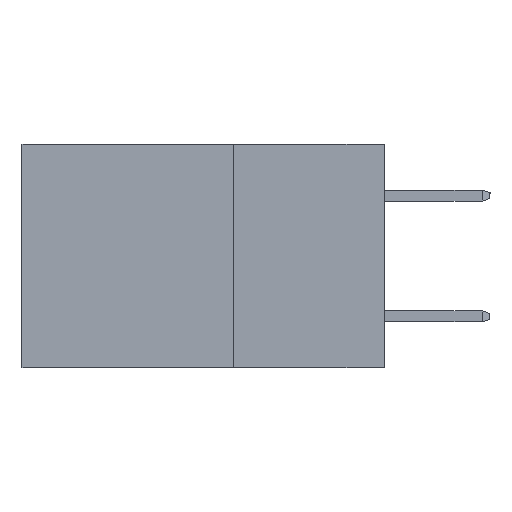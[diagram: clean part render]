
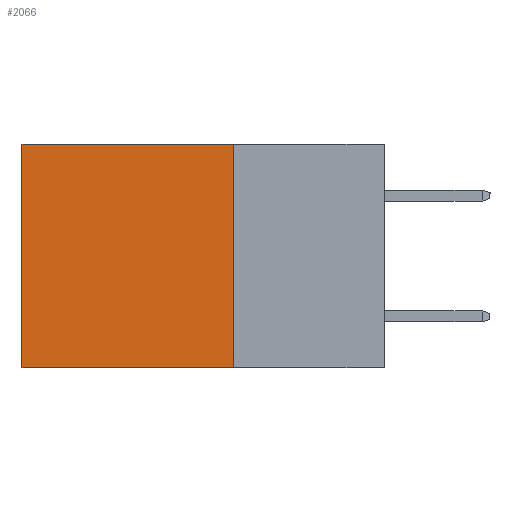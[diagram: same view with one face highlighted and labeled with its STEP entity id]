
A CAD part, left-side view. The second image highlights one B-rep face of the part: STEP entity #2066.
In plain terms, the highlighted planar face has unit normal (-1, 0, 0).
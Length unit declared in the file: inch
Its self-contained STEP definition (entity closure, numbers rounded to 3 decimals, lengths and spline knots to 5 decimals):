
#431 = DIRECTION ( 'NONE',  ( 0., 0., -1. ) ) ;
#452 = AXIS2_PLACEMENT_3D ( 'NONE', #2408, #16525, #431 ) ;
#530 = VERTEX_POINT ( 'NONE', #1109 ) ;
#1109 = CARTESIAN_POINT ( 'NONE',  ( 0.2615, 0.6, 0. ) ) ;
#1752 = ORIENTED_EDGE ( 'NONE', *, *, #14193, .F. ) ;
#2066 = ADVANCED_FACE ( 'NONE', ( #13280 ), #18518, .F. ) ;
#2239 = ORIENTED_EDGE ( 'NONE', *, *, #2568, .T. ) ;
#2408 = CARTESIAN_POINT ( 'NONE',  ( 0.2615, 0.25, -0.37 ) ) ;
#2432 = CARTESIAN_POINT ( 'NONE',  ( 0.2615, 0.25, 0. ) ) ;
#2568 = EDGE_CURVE ( 'NONE', #530, #4409, #3972, .T. ) ;
#3095 = VECTOR ( 'NONE', #10086, 39.37008 ) ;
#3418 = LINE ( 'NONE', #11703, #9938 ) ;
#3870 = LINE ( 'NONE', #7281, #6045 ) ;
#3972 = LINE ( 'NONE', #20282, #5568 ) ;
#4409 = VERTEX_POINT ( 'NONE', #16018 ) ;
#5230 = CARTESIAN_POINT ( 'NONE',  ( 0.2615, 0.25, 0. ) ) ;
#5539 = EDGE_CURVE ( 'NONE', #17838, #14682, #3870, .T. ) ;
#5568 = VECTOR ( 'NONE', #12243, 39.37008 ) ;
#6045 = VECTOR ( 'NONE', #7177, 39.37008 ) ;
#7177 = DIRECTION ( 'NONE',  ( 0., 0., -1. ) ) ;
#7281 = CARTESIAN_POINT ( 'NONE',  ( 0.2615, 0.25, -0.37 ) ) ;
#8036 = DIRECTION ( 'NONE',  ( 0., 1., 0. ) ) ;
#8759 = ORIENTED_EDGE ( 'NONE', *, *, #19135, .T. ) ;
#9938 = VECTOR ( 'NONE', #8036, 39.37008 ) ;
#10048 = CARTESIAN_POINT ( 'NONE',  ( 0.2615, 0.25, -0.37 ) ) ;
#10086 = DIRECTION ( 'NONE',  ( 0., 1., 0. ) ) ;
#11703 = CARTESIAN_POINT ( 'NONE',  ( 0.2615, 0.25, -0.37 ) ) ;
#12243 = DIRECTION ( 'NONE',  ( 0., 0., -1. ) ) ;
#13280 = FACE_OUTER_BOUND ( 'NONE', #19940, .T. ) ;
#14193 = EDGE_CURVE ( 'NONE', #14682, #4409, #3418, .T. ) ;
#14682 = VERTEX_POINT ( 'NONE', #10048 ) ;
#16018 = CARTESIAN_POINT ( 'NONE',  ( 0.2615, 0.6, -0.37 ) ) ;
#16423 = ORIENTED_EDGE ( 'NONE', *, *, #5539, .F. ) ;
#16525 = DIRECTION ( 'NONE',  ( 1., 0., 0. ) ) ;
#17838 = VERTEX_POINT ( 'NONE', #2432 ) ;
#18518 = PLANE ( 'NONE',  #452 ) ;
#19135 = EDGE_CURVE ( 'NONE', #17838, #530, #19723, .T. ) ;
#19723 = LINE ( 'NONE', #5230, #3095 ) ;
#19940 = EDGE_LOOP ( 'NONE', ( #2239, #1752, #16423, #8759 ) ) ;
#20282 = CARTESIAN_POINT ( 'NONE',  ( 0.2615, 0.6, -0.37 ) ) ;
